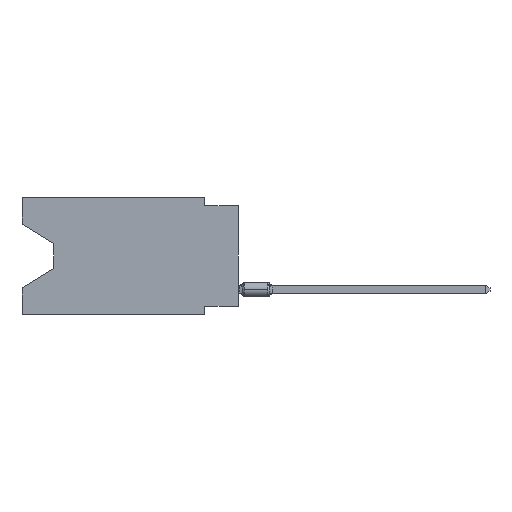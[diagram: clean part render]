
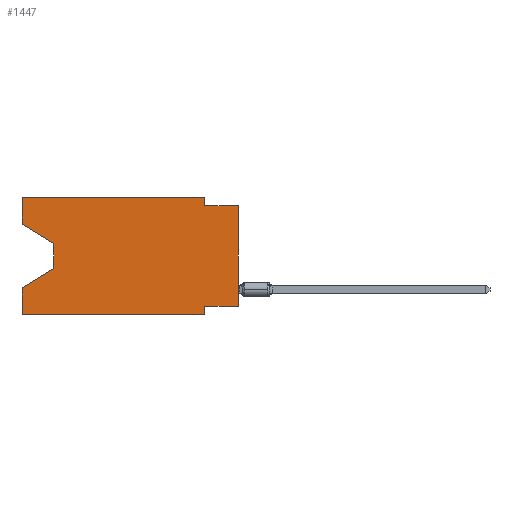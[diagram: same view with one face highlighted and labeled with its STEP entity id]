
A CAD part, left-side view. The second image highlights one B-rep face of the part: STEP entity #1447.
In plain terms, the highlighted planar face has unit normal (-1, 0, 0).
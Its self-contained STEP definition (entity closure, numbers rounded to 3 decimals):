
#648 = CARTESIAN_POINT ( 'NONE',  ( 0., 16.383, -2.038 ) ) ;
#1152 = CARTESIAN_POINT ( 'NONE',  ( 0., 13.97, -5.385 ) ) ;
#1447 = ADVANCED_FACE ( 'NONE', ( #17904 ), #28302, .F. ) ;
#1614 = DIRECTION ( 'NONE',  ( 0., -0.855, -0.519 ) ) ;
#1810 = VECTOR ( 'NONE', #25315, 1000. ) ;
#2182 = EDGE_CURVE ( 'NONE', #26862, #26723, #10498, .T. ) ;
#2540 = ORIENTED_EDGE ( 'NONE', *, *, #21102, .F. ) ;
#2648 = CARTESIAN_POINT ( 'NONE',  ( 0., 2.54, -0.635 ) ) ;
#2700 = VECTOR ( 'NONE', #12273, 1000. ) ;
#2769 = VECTOR ( 'NONE', #22334, 1000. ) ;
#3208 = LINE ( 'NONE', #5507, #2700 ) ;
#3326 = CARTESIAN_POINT ( 'NONE',  ( 0., 2.54, -8.255 ) ) ;
#4007 = DIRECTION ( 'NONE',  ( 0., 0., 1. ) ) ;
#4249 = ORIENTED_EDGE ( 'NONE', *, *, #23463, .T. ) ;
#4624 = DIRECTION ( 'NONE',  ( 0., 0., 1. ) ) ;
#4800 = VERTEX_POINT ( 'NONE', #6759 ) ;
#5122 = VECTOR ( 'NONE', #26345, 1000. ) ;
#5507 = CARTESIAN_POINT ( 'NONE',  ( 0., 16.383, 0. ) ) ;
#5763 = VECTOR ( 'NONE', #1614, 1000. ) ;
#5764 = ORIENTED_EDGE ( 'NONE', *, *, #12533, .F. ) ;
#5918 = ORIENTED_EDGE ( 'NONE', *, *, #22221, .F. ) ;
#6103 = EDGE_CURVE ( 'NONE', #7611, #11816, #14723, .T. ) ;
#6322 = CARTESIAN_POINT ( 'NONE',  ( 0., 2.54, 0. ) ) ;
#6470 = VERTEX_POINT ( 'NONE', #21703 ) ;
#6759 = CARTESIAN_POINT ( 'NONE',  ( 0., 13.97, -3.505 ) ) ;
#7012 = CARTESIAN_POINT ( 'NONE',  ( 0., 13.97, -3.505 ) ) ;
#7075 = LINE ( 'NONE', #15862, #11581 ) ;
#7611 = VERTEX_POINT ( 'NONE', #23488 ) ;
#8062 = EDGE_CURVE ( 'NONE', #26862, #4800, #15332, .T. ) ;
#8300 = LINE ( 'NONE', #19379, #1810 ) ;
#8705 = DIRECTION ( 'NONE',  ( 1., 0., 0. ) ) ;
#8887 = VECTOR ( 'NONE', #27250, 1000. ) ;
#9084 = LINE ( 'NONE', #9218, #2769 ) ;
#9218 = CARTESIAN_POINT ( 'NONE',  ( 0., 0., 0. ) ) ;
#9269 = VECTOR ( 'NONE', #25931, 1000. ) ;
#9307 = LINE ( 'NONE', #7012, #16398 ) ;
#10135 = VERTEX_POINT ( 'NONE', #13585 ) ;
#10414 = CARTESIAN_POINT ( 'NONE',  ( 0., 0., -8.255 ) ) ;
#10498 = LINE ( 'NONE', #25911, #23313 ) ;
#10930 = LINE ( 'NONE', #6322, #24232 ) ;
#11235 = ORIENTED_EDGE ( 'NONE', *, *, #12813, .T. ) ;
#11291 = ORIENTED_EDGE ( 'NONE', *, *, #28123, .T. ) ;
#11346 = DIRECTION ( 'NONE',  ( 0., 0., -1. ) ) ;
#11359 = CARTESIAN_POINT ( 'NONE',  ( 0., 0., -0.635 ) ) ;
#11581 = VECTOR ( 'NONE', #4624, 1000. ) ;
#11816 = VERTEX_POINT ( 'NONE', #3326 ) ;
#12273 = DIRECTION ( 'NONE',  ( 0., -1., 0. ) ) ;
#12533 = EDGE_CURVE ( 'NONE', #6470, #10135, #7075, .T. ) ;
#12813 = EDGE_CURVE ( 'NONE', #20859, #10135, #19290, .T. ) ;
#13585 = CARTESIAN_POINT ( 'NONE',  ( 0., 16.383, -6.852 ) ) ;
#14723 = LINE ( 'NONE', #10414, #5122 ) ;
#14960 = ORIENTED_EDGE ( 'NONE', *, *, #16393, .T. ) ;
#15332 = LINE ( 'NONE', #21496, #5763 ) ;
#15359 = VERTEX_POINT ( 'NONE', #27635 ) ;
#15862 = CARTESIAN_POINT ( 'NONE',  ( 0., 16.383, 0. ) ) ;
#15865 = VERTEX_POINT ( 'NONE', #2648 ) ;
#16284 = ORIENTED_EDGE ( 'NONE', *, *, #2182, .F. ) ;
#16393 = EDGE_CURVE ( 'NONE', #6470, #15359, #26817, .T. ) ;
#16398 = VECTOR ( 'NONE', #11346, 1000. ) ;
#16896 = VERTEX_POINT ( 'NONE', #25213 ) ;
#17478 = CARTESIAN_POINT ( 'NONE',  ( 0., 16.383, 0. ) ) ;
#17904 = FACE_OUTER_BOUND ( 'NONE', #24889, .T. ) ;
#18035 = ORIENTED_EDGE ( 'NONE', *, *, #8062, .T. ) ;
#18954 = ORIENTED_EDGE ( 'NONE', *, *, #24520, .F. ) ;
#19278 = ORIENTED_EDGE ( 'NONE', *, *, #22534, .F. ) ;
#19290 = LINE ( 'NONE', #25651, #9269 ) ;
#19379 = CARTESIAN_POINT ( 'NONE',  ( 0., 2.54, -8.89 ) ) ;
#19705 = DIRECTION ( 'NONE',  ( 0., 0., -1. ) ) ;
#20040 = CARTESIAN_POINT ( 'NONE',  ( 0., 16.383, -8.89 ) ) ;
#20135 = DIRECTION ( 'NONE',  ( 0., -1., 0. ) ) ;
#20859 = VERTEX_POINT ( 'NONE', #1152 ) ;
#21102 = EDGE_CURVE ( 'NONE', #16896, #15865, #10930, .T. ) ;
#21496 = CARTESIAN_POINT ( 'NONE',  ( 0., 16.383, -2.038 ) ) ;
#21703 = CARTESIAN_POINT ( 'NONE',  ( 0., 16.383, -8.89 ) ) ;
#21890 = ORIENTED_EDGE ( 'NONE', *, *, #6103, .F. ) ;
#22221 = EDGE_CURVE ( 'NONE', #15865, #22378, #26629, .T. ) ;
#22334 = DIRECTION ( 'NONE',  ( 0., 0., 1. ) ) ;
#22378 = VERTEX_POINT ( 'NONE', #25191 ) ;
#22534 = EDGE_CURVE ( 'NONE', #11816, #15359, #8300, .T. ) ;
#23313 = VECTOR ( 'NONE', #4007, 1000. ) ;
#23463 = EDGE_CURVE ( 'NONE', #7611, #22378, #9084, .T. ) ;
#23488 = CARTESIAN_POINT ( 'NONE',  ( 0., 0., -8.255 ) ) ;
#24124 = DIRECTION ( 'NONE',  ( 0., 0., -1. ) ) ;
#24232 = VECTOR ( 'NONE', #19705, 1000. ) ;
#24520 = EDGE_CURVE ( 'NONE', #26723, #16896, #3208, .T. ) ;
#24889 = EDGE_LOOP ( 'NONE', ( #18035, #11291, #11235, #5764, #14960, #19278, #21890, #4249, #5918, #2540, #18954, #16284 ) ) ;
#25191 = CARTESIAN_POINT ( 'NONE',  ( 0., 0., -0.635 ) ) ;
#25213 = CARTESIAN_POINT ( 'NONE',  ( 0., 2.54, 0. ) ) ;
#25315 = DIRECTION ( 'NONE',  ( 0., 0., -1. ) ) ;
#25595 = AXIS2_PLACEMENT_3D ( 'NONE', #17478, #8705, #24124 ) ;
#25651 = CARTESIAN_POINT ( 'NONE',  ( 0., 13.97, -5.385 ) ) ;
#25911 = CARTESIAN_POINT ( 'NONE',  ( 0., 16.383, 0. ) ) ;
#25931 = DIRECTION ( 'NONE',  ( 0., 0.855, -0.519 ) ) ;
#26345 = DIRECTION ( 'NONE',  ( 0., 1., 0. ) ) ;
#26629 = LINE ( 'NONE', #11359, #27577 ) ;
#26723 = VERTEX_POINT ( 'NONE', #28465 ) ;
#26817 = LINE ( 'NONE', #20040, #8887 ) ;
#26862 = VERTEX_POINT ( 'NONE', #648 ) ;
#27250 = DIRECTION ( 'NONE',  ( 0., -1., 0. ) ) ;
#27577 = VECTOR ( 'NONE', #20135, 1000. ) ;
#27635 = CARTESIAN_POINT ( 'NONE',  ( 0., 2.54, -8.89 ) ) ;
#28123 = EDGE_CURVE ( 'NONE', #4800, #20859, #9307, .T. ) ;
#28302 = PLANE ( 'NONE',  #25595 ) ;
#28465 = CARTESIAN_POINT ( 'NONE',  ( 0., 16.383, 0. ) ) ;
